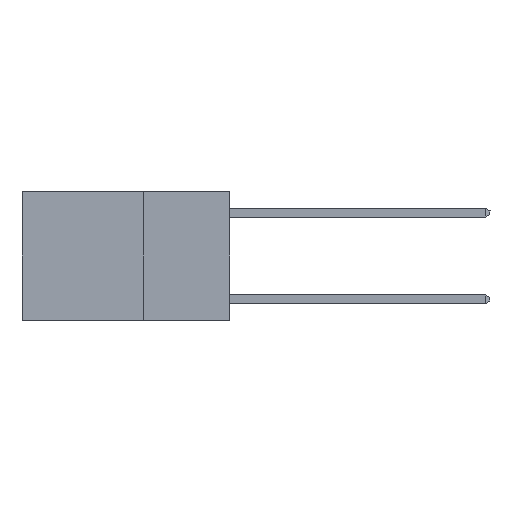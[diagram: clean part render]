
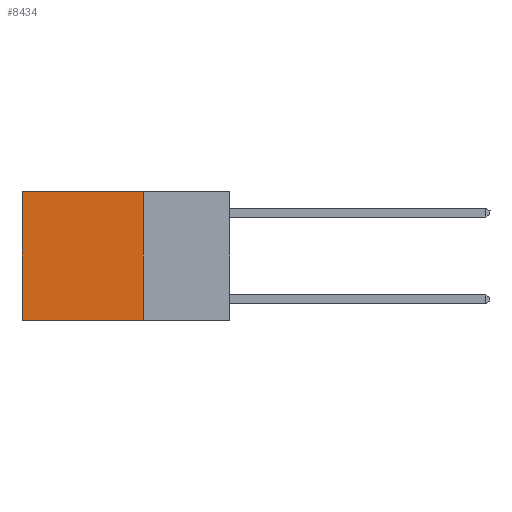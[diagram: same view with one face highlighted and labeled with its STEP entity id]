
A CAD part, left-side view. The second image highlights one B-rep face of the part: STEP entity #8434.
In plain terms, the highlighted planar face has unit normal (-1, 0, 0).
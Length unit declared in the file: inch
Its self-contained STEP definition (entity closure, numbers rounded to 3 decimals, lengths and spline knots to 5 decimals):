
#181 = CARTESIAN_POINT ( 'NONE',  ( 0.2625, 0.25, 0. ) ) ;
#2145 = DIRECTION ( 'NONE',  ( 0., 0., -1. ) ) ;
#2511 = EDGE_CURVE ( 'NONE', #9616, #19085, #7396, .T. ) ;
#3921 = DIRECTION ( 'NONE',  ( 1., 0., 0. ) ) ;
#4183 = PLANE ( 'NONE',  #8444 ) ;
#5013 = VERTEX_POINT ( 'NONE', #15226 ) ;
#5954 = CARTESIAN_POINT ( 'NONE',  ( 0.2625, 0.25, 0. ) ) ;
#6603 = LINE ( 'NONE', #22857, #22905 ) ;
#7396 = LINE ( 'NONE', #18625, #22164 ) ;
#8434 = ADVANCED_FACE ( 'NONE', ( #16841 ), #4183, .F. ) ;
#8444 = AXIS2_PLACEMENT_3D ( 'NONE', #5954, #3921, #2145 ) ;
#8499 = ORIENTED_EDGE ( 'NONE', *, *, #2511, .F. ) ;
#9015 = EDGE_LOOP ( 'NONE', ( #19010, #8499, #16865, #14654 ) ) ;
#9304 = DIRECTION ( 'NONE',  ( 0., 0., -1. ) ) ;
#9616 = VERTEX_POINT ( 'NONE', #16500 ) ;
#10918 = CARTESIAN_POINT ( 'NONE',  ( 0.2625, 0.6, 0. ) ) ;
#11155 = LINE ( 'NONE', #10918, #17181 ) ;
#11981 = VECTOR ( 'NONE', #23513, 39.37008 ) ;
#12575 = LINE ( 'NONE', #181, #11981 ) ;
#13314 = EDGE_CURVE ( 'NONE', #18071, #19085, #11155, .T. ) ;
#13683 = EDGE_CURVE ( 'NONE', #5013, #9616, #6603, .T. ) ;
#14654 = ORIENTED_EDGE ( 'NONE', *, *, #18757, .T. ) ;
#15226 = CARTESIAN_POINT ( 'NONE',  ( 0.2625, 0.25, 0. ) ) ;
#16500 = CARTESIAN_POINT ( 'NONE',  ( 0.2625, 0.25, -0.37 ) ) ;
#16727 = CARTESIAN_POINT ( 'NONE',  ( 0.2625, 0.6, -0.37 ) ) ;
#16775 = DIRECTION ( 'NONE',  ( 0., 1., 0. ) ) ;
#16841 = FACE_OUTER_BOUND ( 'NONE', #9015, .T. ) ;
#16865 = ORIENTED_EDGE ( 'NONE', *, *, #13683, .F. ) ;
#17181 = VECTOR ( 'NONE', #9304, 39.37008 ) ;
#18071 = VERTEX_POINT ( 'NONE', #22835 ) ;
#18625 = CARTESIAN_POINT ( 'NONE',  ( 0.2625, 0.25, -0.37 ) ) ;
#18757 = EDGE_CURVE ( 'NONE', #5013, #18071, #12575, .T. ) ;
#19010 = ORIENTED_EDGE ( 'NONE', *, *, #13314, .T. ) ;
#19085 = VERTEX_POINT ( 'NONE', #16727 ) ;
#21245 = DIRECTION ( 'NONE',  ( 0., 0., -1. ) ) ;
#22164 = VECTOR ( 'NONE', #16775, 39.37008 ) ;
#22835 = CARTESIAN_POINT ( 'NONE',  ( 0.2625, 0.6, 0. ) ) ;
#22857 = CARTESIAN_POINT ( 'NONE',  ( 0.2625, 0.25, 0. ) ) ;
#22905 = VECTOR ( 'NONE', #21245, 39.37008 ) ;
#23513 = DIRECTION ( 'NONE',  ( 0., 1., 0. ) ) ;
